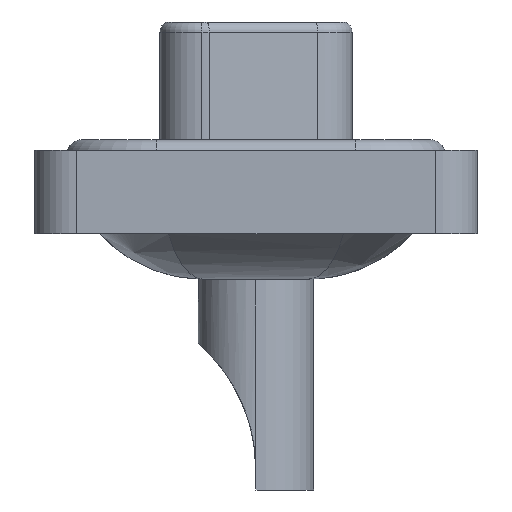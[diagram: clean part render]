
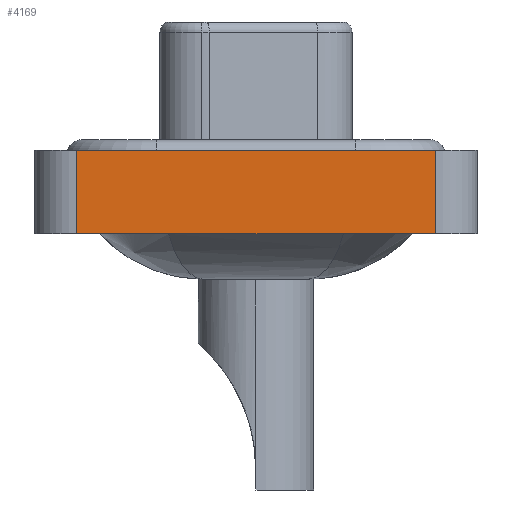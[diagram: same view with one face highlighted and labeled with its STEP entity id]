
A CAD part, left-side view. The second image highlights one B-rep face of the part: STEP entity #4169.
In plain terms, the highlighted planar face has unit normal (-1, 0, 0).
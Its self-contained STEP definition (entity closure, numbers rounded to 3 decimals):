
#663 = VERTEX_POINT ( 'NONE', #6433 ) ;
#1101 = VERTEX_POINT ( 'NONE', #5080 ) ;
#1544 = EDGE_CURVE ( 'NONE', #1101, #9557, #16648, .T. ) ;
#1566 = CARTESIAN_POINT ( 'NONE',  ( -7.3, -8.55, 0.4 ) ) ;
#1606 = CARTESIAN_POINT ( 'NONE',  ( -7.3, 8.55, -3.6 ) ) ;
#4024 = CARTESIAN_POINT ( 'NONE',  ( -7.3, -8.55, -3.6 ) ) ;
#4169 = ADVANCED_FACE ( 'NONE', ( #13261 ), #11695, .T. ) ;
#4236 = ORIENTED_EDGE ( 'NONE', *, *, #13924, .T. ) ;
#4301 = VERTEX_POINT ( 'NONE', #13449 ) ;
#5080 = CARTESIAN_POINT ( 'NONE',  ( -7.3, 8.55, 0.4 ) ) ;
#5206 = EDGE_CURVE ( 'NONE', #663, #1101, #13313, .T. ) ;
#5589 = DIRECTION ( 'NONE',  ( -1., 0., 0. ) ) ;
#5807 = LINE ( 'NONE', #10360, #6817 ) ;
#6433 = CARTESIAN_POINT ( 'NONE',  ( -7.3, 8.55, -3.6 ) ) ;
#6817 = VECTOR ( 'NONE', #7396, 1000. ) ;
#6895 = EDGE_CURVE ( 'NONE', #663, #4301, #8005, .T. ) ;
#7396 = DIRECTION ( 'NONE',  ( 0., 0., 1. ) ) ;
#7648 = VECTOR ( 'NONE', #13713, 1000. ) ;
#7658 = CARTESIAN_POINT ( 'NONE',  ( -7.3, -8.55, 0.4 ) ) ;
#8005 = LINE ( 'NONE', #9583, #9117 ) ;
#8897 = EDGE_LOOP ( 'NONE', ( #4236, #12618, #10826, #9798 ) ) ;
#9117 = VECTOR ( 'NONE', #17218, 1000. ) ;
#9557 = VERTEX_POINT ( 'NONE', #1566 ) ;
#9583 = CARTESIAN_POINT ( 'NONE',  ( -7.3, -8.55, -3.6 ) ) ;
#9798 = ORIENTED_EDGE ( 'NONE', *, *, #6895, .T. ) ;
#10360 = CARTESIAN_POINT ( 'NONE',  ( -7.3, -8.55, -3.6 ) ) ;
#10489 = DIRECTION ( 'NONE',  ( 0., 0., 1. ) ) ;
#10777 = VECTOR ( 'NONE', #10489, 1000. ) ;
#10826 = ORIENTED_EDGE ( 'NONE', *, *, #5206, .F. ) ;
#11695 = PLANE ( 'NONE',  #15769 ) ;
#11886 = DIRECTION ( 'NONE',  ( 0., 0., 1. ) ) ;
#12618 = ORIENTED_EDGE ( 'NONE', *, *, #1544, .F. ) ;
#13261 = FACE_OUTER_BOUND ( 'NONE', #8897, .T. ) ;
#13313 = LINE ( 'NONE', #1606, #10777 ) ;
#13449 = CARTESIAN_POINT ( 'NONE',  ( -7.3, -8.55, -3.6 ) ) ;
#13713 = DIRECTION ( 'NONE',  ( 0., -1., 0. ) ) ;
#13924 = EDGE_CURVE ( 'NONE', #4301, #9557, #5807, .T. ) ;
#15769 = AXIS2_PLACEMENT_3D ( 'NONE', #4024, #5589, #11886 ) ;
#16648 = LINE ( 'NONE', #7658, #7648 ) ;
#17218 = DIRECTION ( 'NONE',  ( 0., -1., 0. ) ) ;
